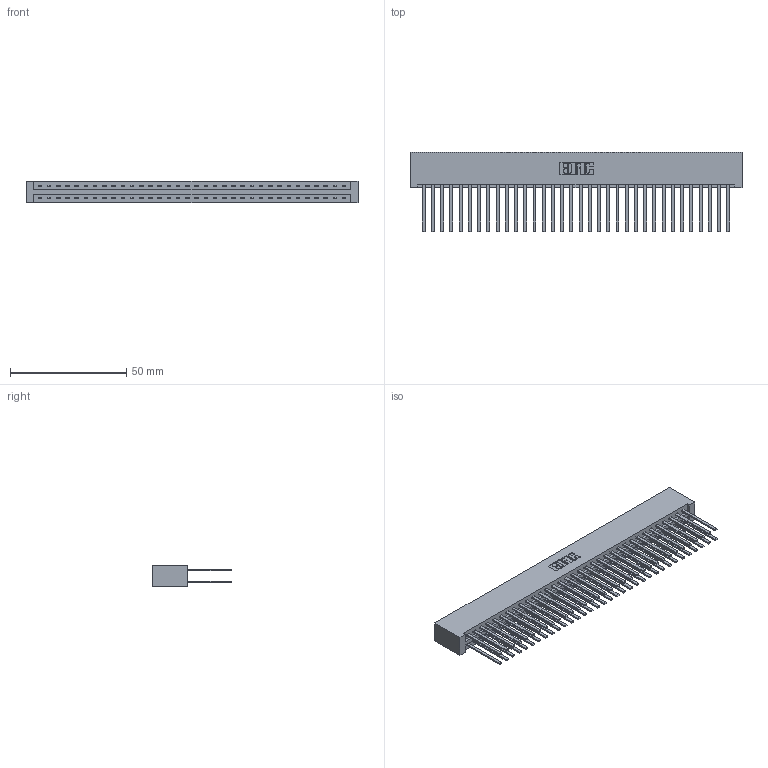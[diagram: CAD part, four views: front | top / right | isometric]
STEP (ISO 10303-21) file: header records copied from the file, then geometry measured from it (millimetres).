
FILE_DESCRIPTION (( 'STEP AP203' ), '1' );
FILE_NAME ('337-068-544-201.STEP', '2018-08-11T10:19:25', ( '' ), ( '' ), 'SwSTEP 2.0', 'SolidWorks 2016', '' );
FILE_SCHEMA (( 'CONFIG_CONTROL_DESIGN' ));
Length unit declared in the file: inch
Products named in the file (3): 337 Part_No Mounting Lugs; 345-292-001_345-293-144; 337-068-544-201
Assembly tree (69 placements, depth 2):
  337-068-544-201
    337 Part_No Mounting Lugs
    345-292-001_345-293-144  x68
Bounding box: 142.6 x 34.3 x 9.4 mm (x, y, z)
Volume: 16635.3 mm3; surface area: 21898.6 mm2
Topology: 69 solids, 69 shells, 3370 faces, 10011 edges, 6582 vertices
Faces by surface type: plane 2378, cylinder 992
Entity records: 26935 total; most frequent: CARTESIAN_POINT 4542, ORIENTED_EDGE 4478, DIRECTION 3867, EDGE_CURVE 2239, LINE 2123, VECTOR 2123, VERTEX_POINT 1490, AXIS2_PLACEMENT_3D 872
